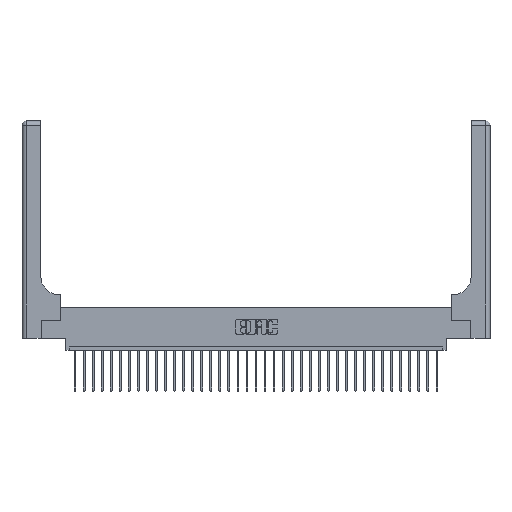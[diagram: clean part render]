
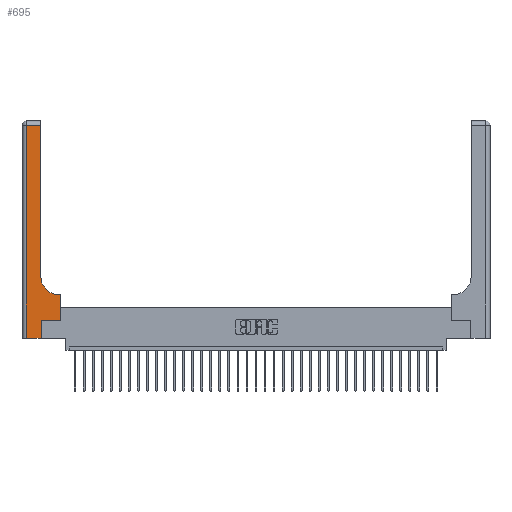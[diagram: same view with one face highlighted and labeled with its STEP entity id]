
A CAD part, top view. The second image highlights one B-rep face of the part: STEP entity #695.
In plain terms, the highlighted planar face has unit normal (0, 0, 1).
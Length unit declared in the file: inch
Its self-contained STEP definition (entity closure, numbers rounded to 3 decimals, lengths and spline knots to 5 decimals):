
#695 = ADVANCED_FACE ( 'NONE', ( #4855 ), #24218, .F. ) ;
#710 = LINE ( 'NONE', #7840, #5157 ) ;
#1069 = ORIENTED_EDGE ( 'NONE', *, *, #1918, .T. ) ;
#1233 = EDGE_CURVE ( 'NONE', #1772, #7372, #11619, .T. ) ;
#1355 = CARTESIAN_POINT ( 'NONE',  ( 0.528, 0.25, 0.37 ) ) ;
#1772 = VERTEX_POINT ( 'NONE', #22871 ) ;
#1918 = EDGE_CURVE ( 'NONE', #7656, #29431, #19505, .T. ) ;
#2142 = VERTEX_POINT ( 'NONE', #30264 ) ;
#2471 = DIRECTION ( 'NONE',  ( 0., 0., -1. ) ) ;
#3567 = VECTOR ( 'NONE', #28007, 39.37008 ) ;
#3584 = ORIENTED_EDGE ( 'NONE', *, *, #23014, .T. ) ;
#4855 = FACE_OUTER_BOUND ( 'NONE', #14876, .T. ) ;
#5024 = AXIS2_PLACEMENT_3D ( 'NONE', #25896, #6383, #11455 ) ;
#5157 = VECTOR ( 'NONE', #10374, 39.37008 ) ;
#5876 = ORIENTED_EDGE ( 'NONE', *, *, #30317, .T. ) ;
#5959 = AXIS2_PLACEMENT_3D ( 'NONE', #28499, #2471, #12158 ) ;
#6383 = DIRECTION ( 'NONE',  ( 0., 0., -1. ) ) ;
#6434 = VERTEX_POINT ( 'NONE', #30484 ) ;
#6629 = CARTESIAN_POINT ( 'NONE',  ( 0.26, 2.94, 0.37 ) ) ;
#6949 = DIRECTION ( 'NONE',  ( 0., 1., 0. ) ) ;
#7102 = CARTESIAN_POINT ( 'NONE',  ( 0.265, 0., 0.37 ) ) ;
#7372 = VERTEX_POINT ( 'NONE', #31028 ) ;
#7656 = VERTEX_POINT ( 'NONE', #18156 ) ;
#7817 = EDGE_CURVE ( 'NONE', #21563, #6434, #26527, .T. ) ;
#7840 = CARTESIAN_POINT ( 'NONE',  ( 0.26, 0.6, 0.37 ) ) ;
#8805 = LINE ( 'NONE', #1355, #3567 ) ;
#9559 = VECTOR ( 'NONE', #9688, 39.37008 ) ;
#9688 = DIRECTION ( 'NONE',  ( -1., 0., 0. ) ) ;
#9990 = CARTESIAN_POINT ( 'NONE',  ( 0., 2.94, 0.37 ) ) ;
#10134 = EDGE_CURVE ( 'NONE', #29431, #18124, #8805, .T. ) ;
#10374 = DIRECTION ( 'NONE',  ( -1., 0., 0. ) ) ;
#11455 = DIRECTION ( 'NONE',  ( 1., 0., 0. ) ) ;
#11619 = LINE ( 'NONE', #25749, #24729 ) ;
#12158 = DIRECTION ( 'NONE',  ( -1., 0., 0. ) ) ;
#12177 = VECTOR ( 'NONE', #12827, 39.37008 ) ;
#12324 = LINE ( 'NONE', #7102, #30391 ) ;
#12650 = ORIENTED_EDGE ( 'NONE', *, *, #1233, .T. ) ;
#12827 = DIRECTION ( 'NONE',  ( 0., 1., 0. ) ) ;
#13773 = VECTOR ( 'NONE', #17940, 39.37008 ) ;
#14876 = EDGE_LOOP ( 'NONE', ( #16923, #29593, #5876, #12650, #3584, #1069, #18854, #15643, #22299 ) ) ;
#14902 = DIRECTION ( 'NONE',  ( 1., 0., 0. ) ) ;
#15643 = ORIENTED_EDGE ( 'NONE', *, *, #24717, .T. ) ;
#16923 = ORIENTED_EDGE ( 'NONE', *, *, #21516, .T. ) ;
#17417 = LINE ( 'NONE', #29630, #12177 ) ;
#17940 = DIRECTION ( 'NONE',  ( 0., -1., 0. ) ) ;
#18124 = VERTEX_POINT ( 'NONE', #28474 ) ;
#18156 = CARTESIAN_POINT ( 'NONE',  ( 0.265, 0.25, 0.37 ) ) ;
#18854 = ORIENTED_EDGE ( 'NONE', *, *, #10134, .T. ) ;
#19505 = LINE ( 'NONE', #22515, #27024 ) ;
#20191 = EDGE_CURVE ( 'NONE', #23619, #2142, #20218, .T. ) ;
#20218 = CIRCLE ( 'NONE', #5024, 0.25 ) ;
#20786 = LINE ( 'NONE', #25398, #13773 ) ;
#21516 = EDGE_CURVE ( 'NONE', #2142, #21563, #17417, .T. ) ;
#21563 = VERTEX_POINT ( 'NONE', #6629 ) ;
#22299 = ORIENTED_EDGE ( 'NONE', *, *, #20191, .T. ) ;
#22515 = CARTESIAN_POINT ( 'NONE',  ( 0.265, 0.25, 0.37 ) ) ;
#22871 = CARTESIAN_POINT ( 'NONE',  ( 0.06, 0., 0.37 ) ) ;
#23014 = EDGE_CURVE ( 'NONE', #7372, #7656, #12324, .T. ) ;
#23619 = VERTEX_POINT ( 'NONE', #29029 ) ;
#24218 = PLANE ( 'NONE',  #5959 ) ;
#24717 = EDGE_CURVE ( 'NONE', #18124, #23619, #710, .T. ) ;
#24729 = VECTOR ( 'NONE', #30338, 39.37008 ) ;
#25398 = CARTESIAN_POINT ( 'NONE',  ( 0.06, 3., 0.37 ) ) ;
#25749 = CARTESIAN_POINT ( 'NONE',  ( 0., 0., 0.37 ) ) ;
#25896 = CARTESIAN_POINT ( 'NONE',  ( 0.51, 0.85, 0.37 ) ) ;
#26527 = LINE ( 'NONE', #9990, #9559 ) ;
#27024 = VECTOR ( 'NONE', #14902, 39.37008 ) ;
#28007 = DIRECTION ( 'NONE',  ( 0., 1., 0. ) ) ;
#28474 = CARTESIAN_POINT ( 'NONE',  ( 0.528, 0.6, 0.37 ) ) ;
#28499 = CARTESIAN_POINT ( 'NONE',  ( 0., 3., 0.37 ) ) ;
#29029 = CARTESIAN_POINT ( 'NONE',  ( 0.51, 0.6, 0.37 ) ) ;
#29431 = VERTEX_POINT ( 'NONE', #30100 ) ;
#29593 = ORIENTED_EDGE ( 'NONE', *, *, #7817, .T. ) ;
#29630 = CARTESIAN_POINT ( 'NONE',  ( 0.26, 3., 0.37 ) ) ;
#30100 = CARTESIAN_POINT ( 'NONE',  ( 0.528, 0.25, 0.37 ) ) ;
#30264 = CARTESIAN_POINT ( 'NONE',  ( 0.26, 0.85, 0.37 ) ) ;
#30317 = EDGE_CURVE ( 'NONE', #6434, #1772, #20786, .T. ) ;
#30338 = DIRECTION ( 'NONE',  ( 1., 0., 0. ) ) ;
#30391 = VECTOR ( 'NONE', #6949, 39.37008 ) ;
#30484 = CARTESIAN_POINT ( 'NONE',  ( 0.06, 2.94, 0.37 ) ) ;
#31028 = CARTESIAN_POINT ( 'NONE',  ( 0.265, 0., 0.37 ) ) ;
